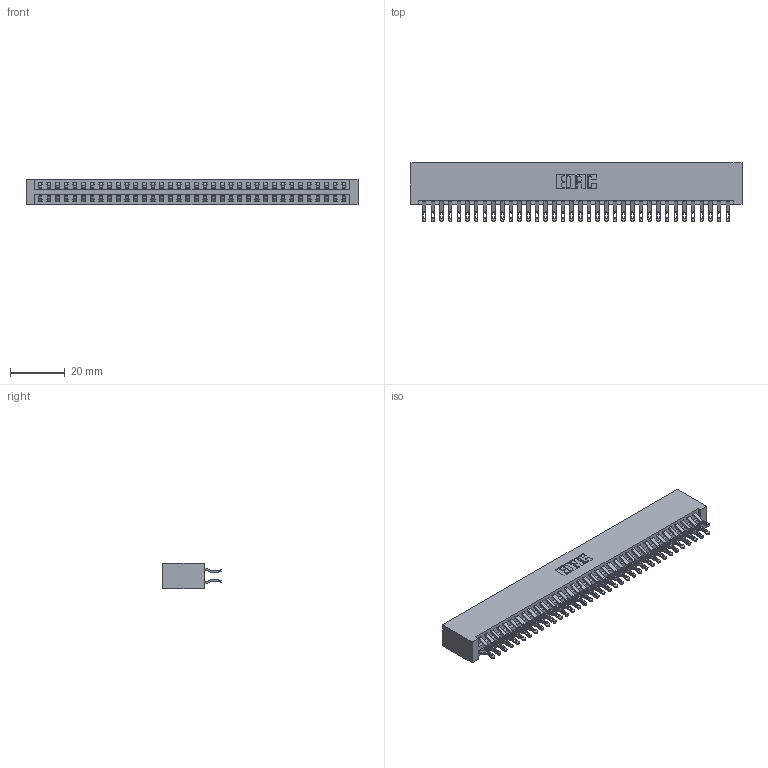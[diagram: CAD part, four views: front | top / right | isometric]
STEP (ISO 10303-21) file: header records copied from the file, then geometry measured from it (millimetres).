
FILE_DESCRIPTION (( 'STEP AP203' ), '1' );
FILE_NAME ('346-072-555-201.STEP', '2018-08-29T01:04:46', ( '' ), ( '' ), 'SwSTEP 2.0', 'SolidWorks 2016', '' );
FILE_SCHEMA (( 'CONFIG_CONTROL_DESIGN' ));
Length unit declared in the file: inch
Products named in the file (3): 346-072-555-201; 346 Part_No Mounting Lugs; 345-292-001_555 Tail
Assembly tree (73 placements, depth 2):
  346-072-555-201
    346 Part_No Mounting Lugs
    345-292-001_555 Tail  x72
Bounding box: 121.54 x 21.46 x 9.4 mm (x, y, z)
Volume: 12587.1 mm3; surface area: 18115.1 mm2
Topology: 73 solids, 73 shells, 4290 faces, 13481 edges, 8986 vertices
Faces by surface type: plane 2448, cylinder 1842
Entity records: 24351 total; most frequent: CARTESIAN_POINT 4054, ORIENTED_EDGE 3958, DIRECTION 3587, EDGE_CURVE 1979, LINE 1691, VECTOR 1691, VERTEX_POINT 1318, AXIS2_PLACEMENT_3D 948
